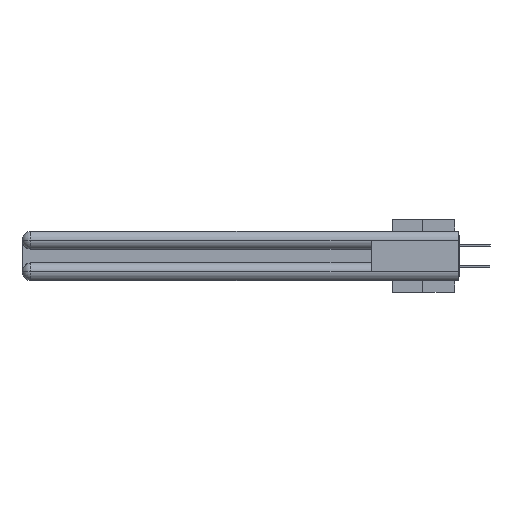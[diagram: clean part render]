
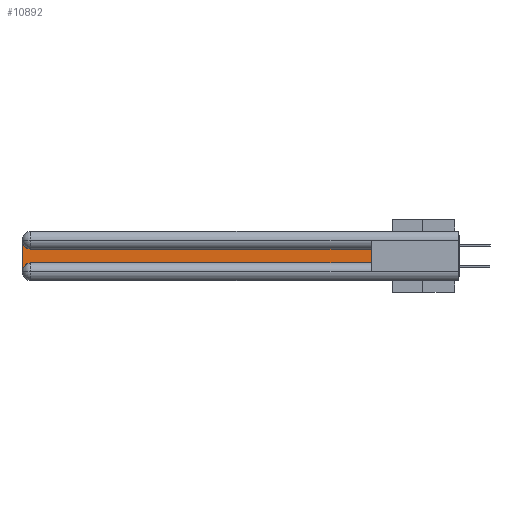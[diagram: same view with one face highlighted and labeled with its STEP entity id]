
A CAD part, left-side view. The second image highlights one B-rep face of the part: STEP entity #10892.
In plain terms, the highlighted planar face has unit normal (-1, 0, 0).
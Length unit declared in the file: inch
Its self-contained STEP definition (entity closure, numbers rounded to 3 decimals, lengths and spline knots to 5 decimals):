
#174 = CARTESIAN_POINT ( 'NONE',  ( 0.075, 0.6, -0.2175 ) ) ;
#201 = VECTOR ( 'NONE', #46536, 39.37008 ) ;
#224 = ORIENTED_EDGE ( 'NONE', *, *, #31896, .T. ) ;
#686 = CARTESIAN_POINT ( 'NONE',  ( 0.075, 2.94, -0.0625 ) ) ;
#1354 = LINE ( 'NONE', #174, #20282 ) ;
#1891 = DIRECTION ( 'NONE',  ( 1., 0., 0. ) ) ;
#2241 = CARTESIAN_POINT ( 'NONE',  ( 0.075, 2.94, -0.1225 ) ) ;
#2531 = CARTESIAN_POINT ( 'NONE',  ( 0.075, 2.94, -0.2175 ) ) ;
#4337 = LINE ( 'NONE', #34253, #18524 ) ;
#5868 = CARTESIAN_POINT ( 'NONE',  ( 0.075, 3., -0.1225 ) ) ;
#6031 = PLANE ( 'NONE',  #43624 ) ;
#6693 = EDGE_CURVE ( 'NONE', #17915, #35320, #4337, .T. ) ;
#9007 = EDGE_CURVE ( 'NONE', #29203, #36558, #1354, .T. ) ;
#9758 = EDGE_CURVE ( 'NONE', #36558, #12857, #39219, .T. ) ;
#10892 = ADVANCED_FACE ( 'NONE', ( #21968 ), #6031, .F. ) ;
#11864 = CARTESIAN_POINT ( 'NONE',  ( 0.075, 0.6, -0.2175 ) ) ;
#12857 = VERTEX_POINT ( 'NONE', #2241 ) ;
#13302 = DIRECTION ( 'NONE',  ( 0., 0., -1. ) ) ;
#17377 = DIRECTION ( 'NONE',  ( 1., 0., 0. ) ) ;
#17915 = VERTEX_POINT ( 'NONE', #43420 ) ;
#18524 = VECTOR ( 'NONE', #26956, 39.37008 ) ;
#18628 = CARTESIAN_POINT ( 'NONE',  ( 0.075, 3., -0.2775 ) ) ;
#19152 = ORIENTED_EDGE ( 'NONE', *, *, #30522, .T. ) ;
#19317 = EDGE_CURVE ( 'NONE', #12857, #17915, #25429, .T. ) ;
#19459 = DIRECTION ( 'NONE',  ( 0., -1., 0. ) ) ;
#20282 = VECTOR ( 'NONE', #33079, 39.37008 ) ;
#21968 = FACE_OUTER_BOUND ( 'NONE', #33899, .T. ) ;
#25429 = CIRCLE ( 'NONE', #39366, 0.06 ) ;
#26342 = CARTESIAN_POINT ( 'NONE',  ( 0.075, 0.6, -0.2175 ) ) ;
#26467 = ORIENTED_EDGE ( 'NONE', *, *, #6693, .T. ) ;
#26956 = DIRECTION ( 'NONE',  ( 0., 0., -1. ) ) ;
#27979 = ORIENTED_EDGE ( 'NONE', *, *, #9007, .T. ) ;
#29203 = VERTEX_POINT ( 'NONE', #26342 ) ;
#29582 = LINE ( 'NONE', #11864, #43844 ) ;
#30522 = EDGE_CURVE ( 'NONE', #35320, #47053, #39732, .T. ) ;
#30816 = AXIS2_PLACEMENT_3D ( 'NONE', #43809, #17377, #36017 ) ;
#31318 = DIRECTION ( 'NONE',  ( 1., 0., 0. ) ) ;
#31896 = EDGE_CURVE ( 'NONE', #47053, #29203, #29582, .T. ) ;
#33079 = DIRECTION ( 'NONE',  ( 0., 0., 1. ) ) ;
#33899 = EDGE_LOOP ( 'NONE', ( #34265, #46531, #26467, #19152, #224, #27979 ) ) ;
#34253 = CARTESIAN_POINT ( 'NONE',  ( 0.075, 3., -0.2175 ) ) ;
#34265 = ORIENTED_EDGE ( 'NONE', *, *, #9758, .T. ) ;
#35320 = VERTEX_POINT ( 'NONE', #18628 ) ;
#35973 = CARTESIAN_POINT ( 'NONE',  ( 0.075, 0.6, -0.1225 ) ) ;
#36017 = DIRECTION ( 'NONE',  ( 0., 0., -1. ) ) ;
#36558 = VERTEX_POINT ( 'NONE', #35973 ) ;
#38172 = DIRECTION ( 'NONE',  ( 0., 0., -1. ) ) ;
#39219 = LINE ( 'NONE', #42136, #201 ) ;
#39366 = AXIS2_PLACEMENT_3D ( 'NONE', #686, #31318, #38172 ) ;
#39732 = CIRCLE ( 'NONE', #30816, 0.06 ) ;
#42136 = CARTESIAN_POINT ( 'NONE',  ( 0.075, 0.6, -0.1225 ) ) ;
#43420 = CARTESIAN_POINT ( 'NONE',  ( 0.075, 3., -0.0625 ) ) ;
#43624 = AXIS2_PLACEMENT_3D ( 'NONE', #5868, #1891, #13302 ) ;
#43809 = CARTESIAN_POINT ( 'NONE',  ( 0.075, 2.94, -0.2775 ) ) ;
#43844 = VECTOR ( 'NONE', #19459, 39.37008 ) ;
#46531 = ORIENTED_EDGE ( 'NONE', *, *, #19317, .T. ) ;
#46536 = DIRECTION ( 'NONE',  ( 0., 1., 0. ) ) ;
#47053 = VERTEX_POINT ( 'NONE', #2531 ) ;
